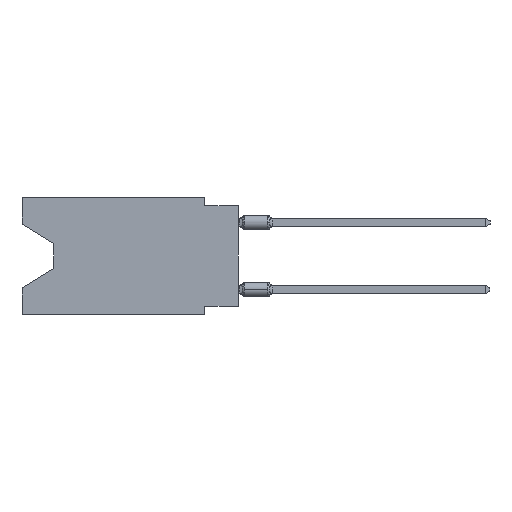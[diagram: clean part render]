
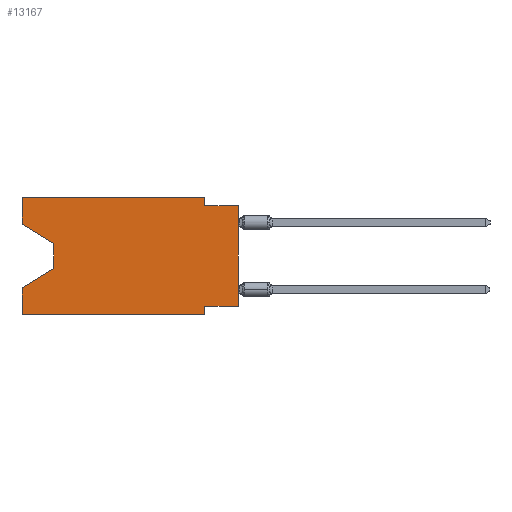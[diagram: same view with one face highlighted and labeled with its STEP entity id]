
A CAD part, left-side view. The second image highlights one B-rep face of the part: STEP entity #13167.
In plain terms, the highlighted planar face has unit normal (-1, 0, 0).
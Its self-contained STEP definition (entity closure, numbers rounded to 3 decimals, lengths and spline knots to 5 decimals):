
#443 = DIRECTION ( 'NONE',  ( 0., -1., 0. ) ) ;
#497 = EDGE_CURVE ( 'NONE', #5940, #4623, #46118, .T. ) ;
#862 = DIRECTION ( 'NONE',  ( 0., 0., 1. ) ) ;
#1700 = CARTESIAN_POINT ( 'NONE',  ( 0., 0., -0.325 ) ) ;
#1982 = CARTESIAN_POINT ( 'NONE',  ( 0., 0., -0.025 ) ) ;
#2111 = CARTESIAN_POINT ( 'NONE',  ( 0., 0.55, -0.212 ) ) ;
#2814 = CARTESIAN_POINT ( 'NONE',  ( 0., 0.55, -0.138 ) ) ;
#2925 = CARTESIAN_POINT ( 'NONE',  ( 0., 0., -0.025 ) ) ;
#3966 = EDGE_CURVE ( 'NONE', #22143, #57844, #54326, .T. ) ;
#4320 = ORIENTED_EDGE ( 'NONE', *, *, #29182, .F. ) ;
#4468 = VECTOR ( 'NONE', #45373, 39.37008 ) ;
#4623 = VERTEX_POINT ( 'NONE', #10310 ) ;
#4667 = CARTESIAN_POINT ( 'NONE',  ( 0., 0.645, 0. ) ) ;
#4849 = EDGE_LOOP ( 'NONE', ( #45097, #30346, #34127, #4320, #25486, #13468, #42482, #44772, #6840, #35565, #8658, #45450 ) ) ;
#4931 = VERTEX_POINT ( 'NONE', #24608 ) ;
#5676 = CARTESIAN_POINT ( 'NONE',  ( 0., 0., 0. ) ) ;
#5686 = DIRECTION ( 'NONE',  ( 0., -1., 0. ) ) ;
#5940 = VERTEX_POINT ( 'NONE', #2814 ) ;
#6380 = VECTOR ( 'NONE', #57157, 39.37008 ) ;
#6615 = DIRECTION ( 'NONE',  ( 0., -0.855, -0.519 ) ) ;
#6840 = ORIENTED_EDGE ( 'NONE', *, *, #3966, .F. ) ;
#7291 = EDGE_CURVE ( 'NONE', #47533, #57844, #10179, .T. ) ;
#7362 = LINE ( 'NONE', #35602, #19268 ) ;
#8658 = ORIENTED_EDGE ( 'NONE', *, *, #42670, .F. ) ;
#9562 = LINE ( 'NONE', #10457, #16922 ) ;
#9888 = CARTESIAN_POINT ( 'NONE',  ( 0., 0.1, -0.325 ) ) ;
#10105 = VECTOR ( 'NONE', #17042, 39.37008 ) ;
#10179 = LINE ( 'NONE', #5676, #42632 ) ;
#10310 = CARTESIAN_POINT ( 'NONE',  ( 0., 0.55, -0.212 ) ) ;
#10457 = CARTESIAN_POINT ( 'NONE',  ( 0., 0.645, 0. ) ) ;
#11983 = VERTEX_POINT ( 'NONE', #45019 ) ;
#12375 = EDGE_CURVE ( 'NONE', #47533, #22579, #51918, .T. ) ;
#13167 = ADVANCED_FACE ( 'NONE', ( #24736 ), #30433, .F. ) ;
#13468 = ORIENTED_EDGE ( 'NONE', *, *, #44161, .F. ) ;
#14466 = VECTOR ( 'NONE', #443, 39.37008 ) ;
#16922 = VECTOR ( 'NONE', #862, 39.37008 ) ;
#17042 = DIRECTION ( 'NONE',  ( 0., -1., 0. ) ) ;
#18583 = EDGE_CURVE ( 'NONE', #4931, #11983, #50686, .T. ) ;
#18725 = CARTESIAN_POINT ( 'NONE',  ( 0., 0.55, -0.138 ) ) ;
#19268 = VECTOR ( 'NONE', #30180, 39.37008 ) ;
#19389 = CARTESIAN_POINT ( 'NONE',  ( 0., 0.645, -0.35 ) ) ;
#19835 = LINE ( 'NONE', #51428, #37855 ) ;
#20020 = DIRECTION ( 'NONE',  ( 0., 1., 0. ) ) ;
#20790 = VECTOR ( 'NONE', #26620, 39.37008 ) ;
#21988 = EDGE_CURVE ( 'NONE', #4623, #22982, #38761, .T. ) ;
#22143 = VERTEX_POINT ( 'NONE', #42316 ) ;
#22452 = CARTESIAN_POINT ( 'NONE',  ( 0., 0.645, -0.26975 ) ) ;
#22579 = VERTEX_POINT ( 'NONE', #9888 ) ;
#22692 = CARTESIAN_POINT ( 'NONE',  ( 0., 0.645, 0. ) ) ;
#22982 = VERTEX_POINT ( 'NONE', #22452 ) ;
#24608 = CARTESIAN_POINT ( 'NONE',  ( 0., 0.645, -0.08025 ) ) ;
#24736 = FACE_OUTER_BOUND ( 'NONE', #4849, .T. ) ;
#24920 = CARTESIAN_POINT ( 'NONE',  ( 0., 0.1, -0.35 ) ) ;
#25486 = ORIENTED_EDGE ( 'NONE', *, *, #36299, .T. ) ;
#26620 = DIRECTION ( 'NONE',  ( 0., 0., 1. ) ) ;
#27016 = LINE ( 'NONE', #35758, #4468 ) ;
#27158 = EDGE_CURVE ( 'NONE', #4931, #5940, #19835, .T. ) ;
#27509 = LINE ( 'NONE', #22692, #14466 ) ;
#29050 = VECTOR ( 'NONE', #41569, 39.37008 ) ;
#29182 = EDGE_CURVE ( 'NONE', #50524, #22982, #9562, .T. ) ;
#30180 = DIRECTION ( 'NONE',  ( 0., 0., -1. ) ) ;
#30346 = ORIENTED_EDGE ( 'NONE', *, *, #497, .T. ) ;
#30433 = PLANE ( 'NONE',  #54114 ) ;
#32289 = CARTESIAN_POINT ( 'NONE',  ( 0., 0.1, 0. ) ) ;
#34127 = ORIENTED_EDGE ( 'NONE', *, *, #21988, .T. ) ;
#35565 = ORIENTED_EDGE ( 'NONE', *, *, #58785, .F. ) ;
#35602 = CARTESIAN_POINT ( 'NONE',  ( 0., 0.1, -0.35 ) ) ;
#35758 = CARTESIAN_POINT ( 'NONE',  ( 0., 0.1, 0. ) ) ;
#36299 = EDGE_CURVE ( 'NONE', #50524, #47467, #46888, .T. ) ;
#37855 = VECTOR ( 'NONE', #6615, 39.37008 ) ;
#38761 = LINE ( 'NONE', #2111, #6380 ) ;
#41569 = DIRECTION ( 'NONE',  ( 0., 0., -1. ) ) ;
#42316 = CARTESIAN_POINT ( 'NONE',  ( 0., 0.1, -0.025 ) ) ;
#42482 = ORIENTED_EDGE ( 'NONE', *, *, #12375, .F. ) ;
#42632 = VECTOR ( 'NONE', #51708, 39.37008 ) ;
#42670 = EDGE_CURVE ( 'NONE', #11983, #48190, #27509, .T. ) ;
#43082 = CARTESIAN_POINT ( 'NONE',  ( 0., 0.645, 0. ) ) ;
#44161 = EDGE_CURVE ( 'NONE', #22579, #47467, #7362, .T. ) ;
#44772 = ORIENTED_EDGE ( 'NONE', *, *, #7291, .T. ) ;
#45019 = CARTESIAN_POINT ( 'NONE',  ( 0., 0.645, 0. ) ) ;
#45097 = ORIENTED_EDGE ( 'NONE', *, *, #27158, .T. ) ;
#45373 = DIRECTION ( 'NONE',  ( 0., 0., -1. ) ) ;
#45450 = ORIENTED_EDGE ( 'NONE', *, *, #18583, .F. ) ;
#46118 = LINE ( 'NONE', #18725, #29050 ) ;
#46888 = LINE ( 'NONE', #55639, #48640 ) ;
#47467 = VERTEX_POINT ( 'NONE', #24920 ) ;
#47533 = VERTEX_POINT ( 'NONE', #56228 ) ;
#48190 = VERTEX_POINT ( 'NONE', #32289 ) ;
#48189 = DIRECTION ( 'NONE',  ( 1., 0., 0. ) ) ;
#48484 = DIRECTION ( 'NONE',  ( 0., 0., -1. ) ) ;
#48640 = VECTOR ( 'NONE', #5686, 39.37008 ) ;
#50524 = VERTEX_POINT ( 'NONE', #19389 ) ;
#50686 = LINE ( 'NONE', #4667, #20790 ) ;
#51428 = CARTESIAN_POINT ( 'NONE',  ( 0., 0.645, -0.08025 ) ) ;
#51708 = DIRECTION ( 'NONE',  ( 0., 0., 1. ) ) ;
#51918 = LINE ( 'NONE', #1700, #59325 ) ;
#54114 = AXIS2_PLACEMENT_3D ( 'NONE', #43082, #48189, #48484 ) ;
#54326 = LINE ( 'NONE', #2925, #10105 ) ;
#55639 = CARTESIAN_POINT ( 'NONE',  ( 0., 0.645, -0.35 ) ) ;
#56228 = CARTESIAN_POINT ( 'NONE',  ( 0., 0., -0.325 ) ) ;
#57157 = DIRECTION ( 'NONE',  ( 0., 0.855, -0.519 ) ) ;
#57844 = VERTEX_POINT ( 'NONE', #1982 ) ;
#58785 = EDGE_CURVE ( 'NONE', #48190, #22143, #27016, .T. ) ;
#59325 = VECTOR ( 'NONE', #20020, 39.37008 ) ;
